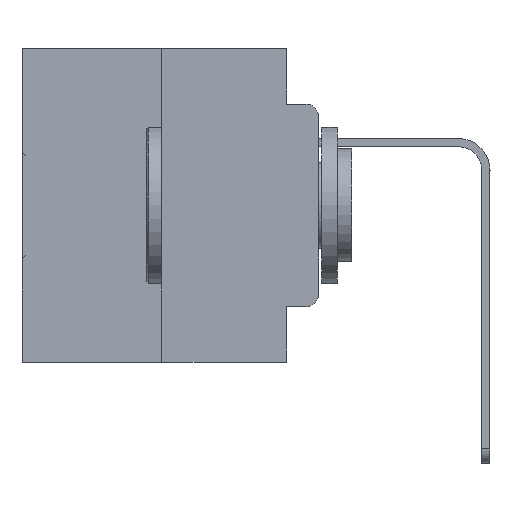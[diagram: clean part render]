
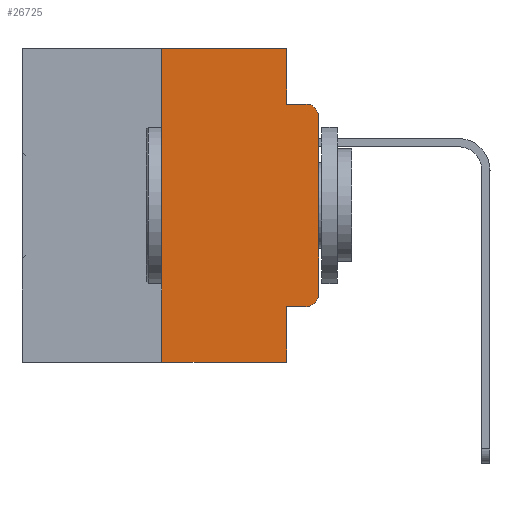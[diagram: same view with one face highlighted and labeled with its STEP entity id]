
A CAD part, left-side view. The second image highlights one B-rep face of the part: STEP entity #26725.
In plain terms, the highlighted planar face has unit normal (-1, 0, 0).
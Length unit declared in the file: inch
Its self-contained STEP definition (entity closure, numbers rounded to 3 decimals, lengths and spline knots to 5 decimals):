
#547 = VECTOR ( 'NONE', #23217, 39.37008 ) ;
#782 = ORIENTED_EDGE ( 'NONE', *, *, #14462, .F. ) ;
#946 = DIRECTION ( 'NONE',  ( 0., -1., 0. ) ) ;
#1299 = PLANE ( 'NONE',  #3117 ) ;
#1572 = VERTEX_POINT ( 'NONE', #11697 ) ;
#1599 = VERTEX_POINT ( 'NONE', #21389 ) ;
#1636 = CARTESIAN_POINT ( 'NONE',  ( 0., 0., -0.3915 ) ) ;
#2245 = VERTEX_POINT ( 'NONE', #20239 ) ;
#2423 = DIRECTION ( 'NONE',  ( 0., 0., -1. ) ) ;
#2531 = VERTEX_POINT ( 'NONE', #1636 ) ;
#2743 = VERTEX_POINT ( 'NONE', #22712 ) ;
#2867 = VECTOR ( 'NONE', #12665, 39.37008 ) ;
#2934 = AXIS2_PLACEMENT_3D ( 'NONE', #13868, #23866, #11943 ) ;
#3117 = AXIS2_PLACEMENT_3D ( 'NONE', #20690, #3703, #20587 ) ;
#3703 = DIRECTION ( 'NONE',  ( 1., 0., 0. ) ) ;
#3745 = VECTOR ( 'NONE', #2423, 39.37008 ) ;
#4023 = DIRECTION ( 'NONE',  ( 0., -1., 0. ) ) ;
#4204 = CARTESIAN_POINT ( 'NONE',  ( 0., 0.473, -0.5 ) ) ;
#4669 = DIRECTION ( 'NONE',  ( 0., 0., -1. ) ) ;
#6638 = LINE ( 'NONE', #19712, #2867 ) ;
#6770 = ORIENTED_EDGE ( 'NONE', *, *, #11400, .T. ) ;
#7302 = CARTESIAN_POINT ( 'NONE',  ( 0., 0.051, 0. ) ) ;
#7669 = EDGE_CURVE ( 'NONE', #14129, #1572, #25816, .T. ) ;
#8060 = CARTESIAN_POINT ( 'NONE',  ( 0., 0.051, -0.4115 ) ) ;
#8846 = CARTESIAN_POINT ( 'NONE',  ( 0., 0., -0.1085 ) ) ;
#9460 = EDGE_LOOP ( 'NONE', ( #14450, #27483, #25015, #15082, #17854, #28847, #24685, #782, #6770, #11209 ) ) ;
#9486 = LINE ( 'NONE', #7302, #3745 ) ;
#9493 = CARTESIAN_POINT ( 'NONE',  ( 0., 0.051, 0. ) ) ;
#9697 = VECTOR ( 'NONE', #13431, 39.37008 ) ;
#10565 = CARTESIAN_POINT ( 'NONE',  ( 0., 0.25, -0.5 ) ) ;
#10573 = VERTEX_POINT ( 'NONE', #8846 ) ;
#11209 = ORIENTED_EDGE ( 'NONE', *, *, #18193, .T. ) ;
#11400 = EDGE_CURVE ( 'NONE', #1599, #2743, #24373, .T. ) ;
#11692 = DIRECTION ( 'NONE',  ( 0., -1., 0. ) ) ;
#11697 = CARTESIAN_POINT ( 'NONE',  ( 0., 0.25, 0. ) ) ;
#11706 = CARTESIAN_POINT ( 'NONE',  ( 0., 0.473, 0. ) ) ;
#11943 = DIRECTION ( 'NONE',  ( 0., 0., -1. ) ) ;
#12665 = DIRECTION ( 'NONE',  ( 0., -1., 0. ) ) ;
#13408 = CARTESIAN_POINT ( 'NONE',  ( 0., 0.051, -0.5 ) ) ;
#13431 = DIRECTION ( 'NONE',  ( 0., 0., -1. ) ) ;
#13868 = CARTESIAN_POINT ( 'NONE',  ( 0., 0.02, -0.3915 ) ) ;
#14129 = VERTEX_POINT ( 'NONE', #10565 ) ;
#14450 = ORIENTED_EDGE ( 'NONE', *, *, #30651, .T. ) ;
#14462 = EDGE_CURVE ( 'NONE', #1599, #18742, #9486, .T. ) ;
#14951 = VECTOR ( 'NONE', #946, 39.37008 ) ;
#15082 = ORIENTED_EDGE ( 'NONE', *, *, #26669, .F. ) ;
#16758 = DIRECTION ( 'NONE',  ( 0., 0., 1. ) ) ;
#17443 = CARTESIAN_POINT ( 'NONE',  ( 0., 0.051, 0. ) ) ;
#17629 = CIRCLE ( 'NONE', #22148, 0.02 ) ;
#17854 = ORIENTED_EDGE ( 'NONE', *, *, #26927, .F. ) ;
#18193 = EDGE_CURVE ( 'NONE', #2743, #2531, #29767, .T. ) ;
#18742 = VERTEX_POINT ( 'NONE', #13408 ) ;
#19052 = EDGE_CURVE ( 'NONE', #10573, #2245, #17629, .T. ) ;
#19712 = CARTESIAN_POINT ( 'NONE',  ( 0., 0.051, -0.0885 ) ) ;
#19870 = EDGE_CURVE ( 'NONE', #20497, #2245, #6638, .T. ) ;
#20224 = LINE ( 'NONE', #11706, #30038 ) ;
#20236 = FACE_OUTER_BOUND ( 'NONE', #9460, .T. ) ;
#20239 = CARTESIAN_POINT ( 'NONE',  ( 0., 0.02, -0.0885 ) ) ;
#20497 = VERTEX_POINT ( 'NONE', #22945 ) ;
#20587 = DIRECTION ( 'NONE',  ( 0., 0., -1. ) ) ;
#20690 = CARTESIAN_POINT ( 'NONE',  ( 0., 0.473, 0. ) ) ;
#21389 = CARTESIAN_POINT ( 'NONE',  ( 0., 0.051, -0.4115 ) ) ;
#21437 = CARTESIAN_POINT ( 'NONE',  ( 0., 0.02, -0.1085 ) ) ;
#21747 = LINE ( 'NONE', #17443, #9697 ) ;
#22148 = AXIS2_PLACEMENT_3D ( 'NONE', #21437, #28746, #4669 ) ;
#22712 = CARTESIAN_POINT ( 'NONE',  ( 0., 0.02, -0.4115 ) ) ;
#22945 = CARTESIAN_POINT ( 'NONE',  ( 0., 0.051, -0.0885 ) ) ;
#23217 = DIRECTION ( 'NONE',  ( 0., 0., 1. ) ) ;
#23510 = EDGE_CURVE ( 'NONE', #14129, #18742, #24965, .T. ) ;
#23563 = VERTEX_POINT ( 'NONE', #9493 ) ;
#23612 = CARTESIAN_POINT ( 'NONE',  ( 0., 0., 0. ) ) ;
#23866 = DIRECTION ( 'NONE',  ( -1., 0., 0. ) ) ;
#23994 = LINE ( 'NONE', #23612, #28908 ) ;
#24205 = VECTOR ( 'NONE', #11692, 39.37008 ) ;
#24373 = LINE ( 'NONE', #8060, #14951 ) ;
#24685 = ORIENTED_EDGE ( 'NONE', *, *, #23510, .T. ) ;
#24965 = LINE ( 'NONE', #4204, #24205 ) ;
#25015 = ORIENTED_EDGE ( 'NONE', *, *, #19870, .F. ) ;
#25816 = LINE ( 'NONE', #27986, #547 ) ;
#26669 = EDGE_CURVE ( 'NONE', #23563, #20497, #21747, .T. ) ;
#26725 = ADVANCED_FACE ( 'NONE', ( #20236 ), #1299, .F. ) ;
#26927 = EDGE_CURVE ( 'NONE', #1572, #23563, #20224, .T. ) ;
#27483 = ORIENTED_EDGE ( 'NONE', *, *, #19052, .T. ) ;
#27986 = CARTESIAN_POINT ( 'NONE',  ( 0., 0.25, 0. ) ) ;
#28746 = DIRECTION ( 'NONE',  ( -1., 0., 0. ) ) ;
#28847 = ORIENTED_EDGE ( 'NONE', *, *, #7669, .F. ) ;
#28908 = VECTOR ( 'NONE', #16758, 39.37008 ) ;
#29767 = CIRCLE ( 'NONE', #2934, 0.02 ) ;
#30038 = VECTOR ( 'NONE', #4023, 39.37008 ) ;
#30651 = EDGE_CURVE ( 'NONE', #2531, #10573, #23994, .T. ) ;
